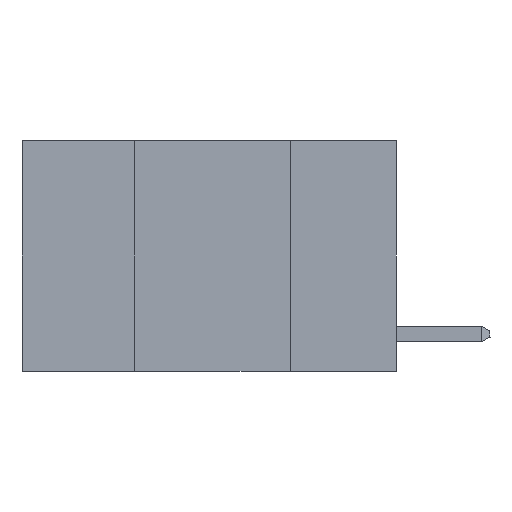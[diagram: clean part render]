
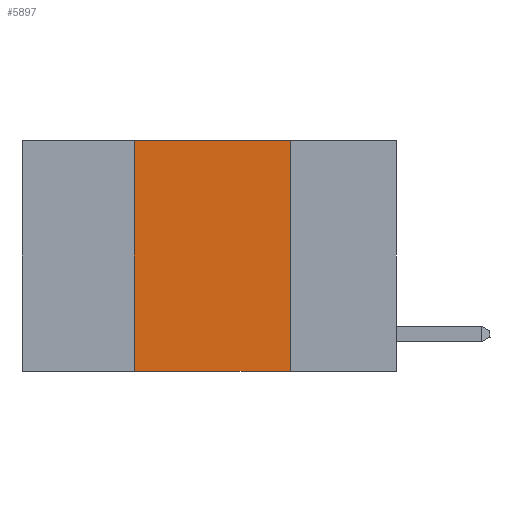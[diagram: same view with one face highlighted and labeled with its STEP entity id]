
A CAD part, left-side view. The second image highlights one B-rep face of the part: STEP entity #5897.
In plain terms, the highlighted planar face has unit normal (-1, 0, 0).
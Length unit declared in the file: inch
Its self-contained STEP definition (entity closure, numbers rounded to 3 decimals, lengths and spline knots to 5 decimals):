
#746 = EDGE_CURVE ( 'NONE', #1786, #5748, #4303, .T. ) ;
#873 = LINE ( 'NONE', #6020, #3812 ) ;
#1059 = DIRECTION ( 'NONE',  ( 0., 0., -1. ) ) ;
#1380 = VECTOR ( 'NONE', #3122, 39.37008 ) ;
#1740 = EDGE_CURVE ( 'NONE', #10885, #5748, #4145, .T. ) ;
#1786 = VERTEX_POINT ( 'NONE', #11385 ) ;
#1792 = EDGE_CURVE ( 'NONE', #5907, #1786, #873, .T. ) ;
#2954 = DIRECTION ( 'NONE',  ( 0., 0., 1. ) ) ;
#2971 = CARTESIAN_POINT ( 'NONE',  ( 0., 0.17, -0.37 ) ) ;
#3122 = DIRECTION ( 'NONE',  ( 0., 0., -1. ) ) ;
#3281 = ORIENTED_EDGE ( 'NONE', *, *, #746, .F. ) ;
#3501 = CARTESIAN_POINT ( 'NONE',  ( 0., 0.17, 0. ) ) ;
#3812 = VECTOR ( 'NONE', #13412, 39.37008 ) ;
#4145 = LINE ( 'NONE', #7085, #12298 ) ;
#4303 = LINE ( 'NONE', #3501, #1380 ) ;
#4355 = CARTESIAN_POINT ( 'NONE',  ( 0., 0.42, 0. ) ) ;
#5748 = VERTEX_POINT ( 'NONE', #2971 ) ;
#5897 = ADVANCED_FACE ( 'NONE', ( #8757 ), #13815, .F. ) ;
#5907 = VERTEX_POINT ( 'NONE', #4355 ) ;
#6020 = CARTESIAN_POINT ( 'NONE',  ( 0., 0.6, 0. ) ) ;
#6197 = EDGE_LOOP ( 'NONE', ( #3281, #12699, #13470, #6415 ) ) ;
#6415 = ORIENTED_EDGE ( 'NONE', *, *, #1740, .T. ) ;
#7085 = CARTESIAN_POINT ( 'NONE',  ( 0., 0.6, -0.37 ) ) ;
#7474 = AXIS2_PLACEMENT_3D ( 'NONE', #11785, #7613, #1059 ) ;
#7613 = DIRECTION ( 'NONE',  ( 1., 0., 0. ) ) ;
#8331 = EDGE_CURVE ( 'NONE', #10885, #5907, #12740, .T. ) ;
#8757 = FACE_OUTER_BOUND ( 'NONE', #6197, .T. ) ;
#9025 = VECTOR ( 'NONE', #2954, 39.37008 ) ;
#9036 = CARTESIAN_POINT ( 'NONE',  ( 0., 0.42, -0.37 ) ) ;
#9153 = DIRECTION ( 'NONE',  ( 0., -1., 0. ) ) ;
#9462 = CARTESIAN_POINT ( 'NONE',  ( 0., 0.42, 0. ) ) ;
#10885 = VERTEX_POINT ( 'NONE', #9036 ) ;
#11385 = CARTESIAN_POINT ( 'NONE',  ( 0., 0.17, 0. ) ) ;
#11785 = CARTESIAN_POINT ( 'NONE',  ( 0., 0.6, 0. ) ) ;
#12298 = VECTOR ( 'NONE', #9153, 39.37008 ) ;
#12699 = ORIENTED_EDGE ( 'NONE', *, *, #1792, .F. ) ;
#12740 = LINE ( 'NONE', #9462, #9025 ) ;
#13412 = DIRECTION ( 'NONE',  ( 0., -1., 0. ) ) ;
#13470 = ORIENTED_EDGE ( 'NONE', *, *, #8331, .F. ) ;
#13815 = PLANE ( 'NONE',  #7474 ) ;
